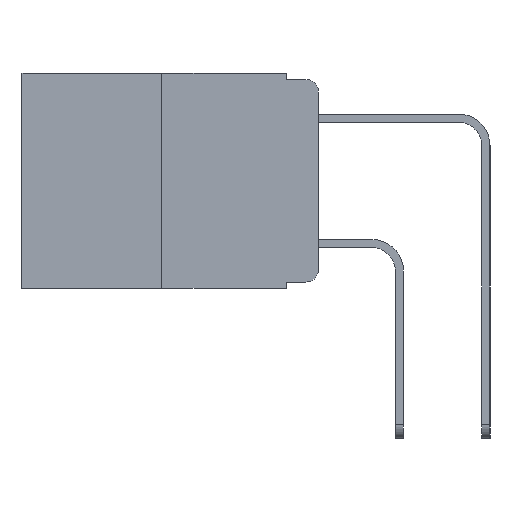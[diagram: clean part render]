
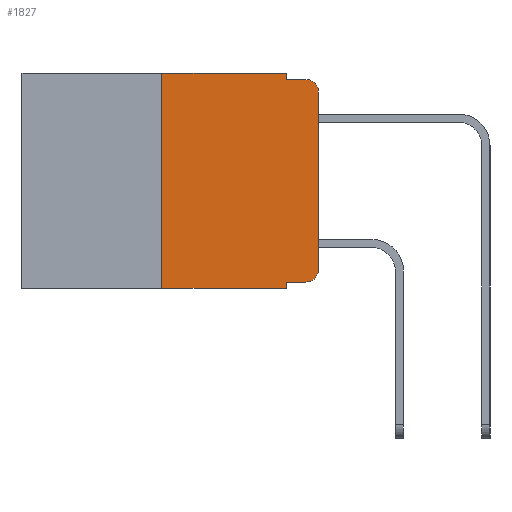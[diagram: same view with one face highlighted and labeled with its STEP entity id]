
A CAD part, left-side view. The second image highlights one B-rep face of the part: STEP entity #1827.
In plain terms, the highlighted planar face has unit normal (-1, 0, 0).
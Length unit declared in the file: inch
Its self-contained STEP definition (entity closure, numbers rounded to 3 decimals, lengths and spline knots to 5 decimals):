
#515 = EDGE_CURVE ( 'NONE', #8627, #8024, #12384, .T. ) ;
#690 = CARTESIAN_POINT ( 'NONE',  ( 0., 0.051, -0.333 ) ) ;
#936 = DIRECTION ( 'NONE',  ( 0., 0., -1. ) ) ;
#1162 = VERTEX_POINT ( 'NONE', #690 ) ;
#1371 = CARTESIAN_POINT ( 'NONE',  ( 0., 0.473, 0. ) ) ;
#1655 = VECTOR ( 'NONE', #8020, 39.37008 ) ;
#1683 = EDGE_CURVE ( 'NONE', #1162, #8024, #9430, .T. ) ;
#1799 = VECTOR ( 'NONE', #2330, 39.37008 ) ;
#1827 = ADVANCED_FACE ( 'NONE', ( #10755 ), #6835, .F. ) ;
#1973 = LINE ( 'NONE', #10762, #4596 ) ;
#2183 = CARTESIAN_POINT ( 'NONE',  ( 0., 0.051, 0. ) ) ;
#2258 = DIRECTION ( 'NONE',  ( 0., 0., 1. ) ) ;
#2302 = CARTESIAN_POINT ( 'NONE',  ( 0., 0.051, -0.01 ) ) ;
#2330 = DIRECTION ( 'NONE',  ( 0., 0., -1. ) ) ;
#3017 = DIRECTION ( 'NONE',  ( 0., -1., 0. ) ) ;
#3264 = EDGE_CURVE ( 'NONE', #1162, #8932, #7811, .T. ) ;
#3311 = CARTESIAN_POINT ( 'NONE',  ( 0., 0.02, -0.01 ) ) ;
#3519 = CARTESIAN_POINT ( 'NONE',  ( 0., 0., 0. ) ) ;
#3864 = DIRECTION ( 'NONE',  ( 0., -1., 0. ) ) ;
#3994 = DIRECTION ( 'NONE',  ( 0., -1., 0. ) ) ;
#4278 = EDGE_LOOP ( 'NONE', ( #9743, #8981, #9238, #9423, #9078, #9283, #9446, #9663, #6612, #9675 ) ) ;
#4427 = LINE ( 'NONE', #5244, #1799 ) ;
#4500 = DIRECTION ( 'NONE',  ( 0., 0., 1. ) ) ;
#4596 = VECTOR ( 'NONE', #2258, 39.37008 ) ;
#4672 = AXIS2_PLACEMENT_3D ( 'NONE', #5324, #11860, #6261 ) ;
#5156 = CARTESIAN_POINT ( 'NONE',  ( 0., 0.25, 0. ) ) ;
#5180 = DIRECTION ( 'NONE',  ( 1., 0., 0. ) ) ;
#5200 = LINE ( 'NONE', #2302, #1655 ) ;
#5244 = CARTESIAN_POINT ( 'NONE',  ( 0., 0.051, 0. ) ) ;
#5324 = CARTESIAN_POINT ( 'NONE',  ( 0., 0.02, -0.03 ) ) ;
#5535 = EDGE_CURVE ( 'NONE', #7873, #9516, #9751, .T. ) ;
#6254 = EDGE_CURVE ( 'NONE', #8627, #7873, #1973, .T. ) ;
#6261 = DIRECTION ( 'NONE',  ( 0., 0., -1. ) ) ;
#6278 = EDGE_CURVE ( 'NONE', #12077, #6282, #5200, .T. ) ;
#6282 = VERTEX_POINT ( 'NONE', #3311 ) ;
#6311 = CARTESIAN_POINT ( 'NONE',  ( 0., 0.051, -0.343 ) ) ;
#6612 = ORIENTED_EDGE ( 'NONE', *, *, #3264, .T. ) ;
#6780 = DIRECTION ( 'NONE',  ( -1., 0., 0. ) ) ;
#6835 = PLANE ( 'NONE',  #9246 ) ;
#6864 = VECTOR ( 'NONE', #3864, 39.37008 ) ;
#6891 = EDGE_CURVE ( 'NONE', #9516, #12077, #4427, .T. ) ;
#6933 = VERTEX_POINT ( 'NONE', #11872 ) ;
#6990 = VECTOR ( 'NONE', #10149, 39.37008 ) ;
#7265 = EDGE_CURVE ( 'NONE', #8932, #11999, #8355, .T. ) ;
#7291 = CARTESIAN_POINT ( 'NONE',  ( 0., 0.25, -0.343 ) ) ;
#7553 = CARTESIAN_POINT ( 'NONE',  ( 0., 0., -0.313 ) ) ;
#7662 = CARTESIAN_POINT ( 'NONE',  ( 0., 0.02, -0.333 ) ) ;
#7811 = LINE ( 'NONE', #8411, #10005 ) ;
#7873 = VERTEX_POINT ( 'NONE', #5156 ) ;
#8020 = DIRECTION ( 'NONE',  ( 0., -1., 0. ) ) ;
#8024 = VERTEX_POINT ( 'NONE', #6311 ) ;
#8355 = CIRCLE ( 'NONE', #10465, 0.02 ) ;
#8411 = CARTESIAN_POINT ( 'NONE',  ( 0., 0.051, -0.333 ) ) ;
#8627 = VERTEX_POINT ( 'NONE', #7291 ) ;
#8932 = VERTEX_POINT ( 'NONE', #7662 ) ;
#8981 = ORIENTED_EDGE ( 'NONE', *, *, #9995, .T. ) ;
#9048 = VECTOR ( 'NONE', #4500, 39.37008 ) ;
#9078 = ORIENTED_EDGE ( 'NONE', *, *, #5535, .F. ) ;
#9238 = ORIENTED_EDGE ( 'NONE', *, *, #6278, .F. ) ;
#9246 = AXIS2_PLACEMENT_3D ( 'NONE', #1371, #5180, #11732 ) ;
#9283 = ORIENTED_EDGE ( 'NONE', *, *, #6254, .F. ) ;
#9330 = LINE ( 'NONE', #3519, #9048 ) ;
#9423 = ORIENTED_EDGE ( 'NONE', *, *, #6891, .F. ) ;
#9430 = LINE ( 'NONE', #2183, #6990 ) ;
#9433 = VECTOR ( 'NONE', #3017, 39.37008 ) ;
#9446 = ORIENTED_EDGE ( 'NONE', *, *, #515, .T. ) ;
#9516 = VERTEX_POINT ( 'NONE', #10462 ) ;
#9663 = ORIENTED_EDGE ( 'NONE', *, *, #1683, .F. ) ;
#9675 = ORIENTED_EDGE ( 'NONE', *, *, #7265, .T. ) ;
#9743 = ORIENTED_EDGE ( 'NONE', *, *, #10716, .T. ) ;
#9751 = LINE ( 'NONE', #10575, #9433 ) ;
#9924 = CIRCLE ( 'NONE', #4672, 0.02 ) ;
#9995 = EDGE_CURVE ( 'NONE', #6933, #6282, #9924, .T. ) ;
#10005 = VECTOR ( 'NONE', #3994, 39.37008 ) ;
#10149 = DIRECTION ( 'NONE',  ( 0., 0., -1. ) ) ;
#10462 = CARTESIAN_POINT ( 'NONE',  ( 0., 0.051, 0. ) ) ;
#10465 = AXIS2_PLACEMENT_3D ( 'NONE', #12345, #6780, #936 ) ;
#10486 = CARTESIAN_POINT ( 'NONE',  ( 0., 0.051, -0.01 ) ) ;
#10538 = CARTESIAN_POINT ( 'NONE',  ( 0., 0.473, -0.343 ) ) ;
#10575 = CARTESIAN_POINT ( 'NONE',  ( 0., 0.473, 0. ) ) ;
#10716 = EDGE_CURVE ( 'NONE', #11999, #6933, #9330, .T. ) ;
#10755 = FACE_OUTER_BOUND ( 'NONE', #4278, .T. ) ;
#10762 = CARTESIAN_POINT ( 'NONE',  ( 0., 0.25, 0. ) ) ;
#11732 = DIRECTION ( 'NONE',  ( 0., 0., -1. ) ) ;
#11860 = DIRECTION ( 'NONE',  ( -1., 0., 0. ) ) ;
#11872 = CARTESIAN_POINT ( 'NONE',  ( 0., 0., -0.03 ) ) ;
#11999 = VERTEX_POINT ( 'NONE', #7553 ) ;
#12077 = VERTEX_POINT ( 'NONE', #10486 ) ;
#12345 = CARTESIAN_POINT ( 'NONE',  ( 0., 0.02, -0.313 ) ) ;
#12384 = LINE ( 'NONE', #10538, #6864 ) ;
